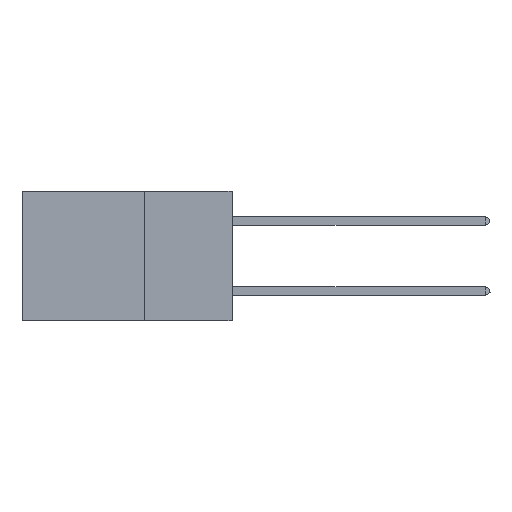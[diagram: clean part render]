
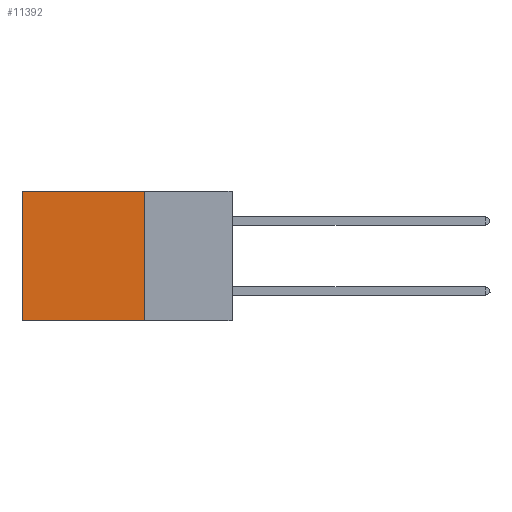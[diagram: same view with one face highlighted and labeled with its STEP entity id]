
A CAD part, left-side view. The second image highlights one B-rep face of the part: STEP entity #11392.
In plain terms, the highlighted planar face has unit normal (-1, 0, 0).
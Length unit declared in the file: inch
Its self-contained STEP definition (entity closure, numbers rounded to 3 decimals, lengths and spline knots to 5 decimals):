
#545 = CARTESIAN_POINT ( 'NONE',  ( 0.2875, 0.6, 0. ) ) ;
#556 = VERTEX_POINT ( 'NONE', #7631 ) ;
#778 = ORIENTED_EDGE ( 'NONE', *, *, #7028, .F. ) ;
#787 = EDGE_CURVE ( 'NONE', #556, #21670, #19484, .T. ) ;
#1865 = EDGE_CURVE ( 'NONE', #556, #8646, #19161, .T. ) ;
#1885 = VECTOR ( 'NONE', #12002, 39.37008 ) ;
#2304 = VERTEX_POINT ( 'NONE', #20187 ) ;
#3359 = AXIS2_PLACEMENT_3D ( 'NONE', #5498, #18232, #27047 ) ;
#5120 = EDGE_LOOP ( 'NONE', ( #17903, #778, #9570, #25273 ) ) ;
#5498 = CARTESIAN_POINT ( 'NONE',  ( 0.2875, 0.25, 0. ) ) ;
#7028 = EDGE_CURVE ( 'NONE', #8646, #2304, #26189, .T. ) ;
#7631 = CARTESIAN_POINT ( 'NONE',  ( 0.2875, 0.25, 0. ) ) ;
#7740 = VECTOR ( 'NONE', #9291, 39.37008 ) ;
#8248 = EDGE_CURVE ( 'NONE', #21670, #2304, #11084, .T. ) ;
#8646 = VERTEX_POINT ( 'NONE', #10606 ) ;
#9291 = DIRECTION ( 'NONE',  ( 0., 0., -1. ) ) ;
#9570 = ORIENTED_EDGE ( 'NONE', *, *, #1865, .F. ) ;
#10003 = CARTESIAN_POINT ( 'NONE',  ( 0.2875, 0.25, 0. ) ) ;
#10606 = CARTESIAN_POINT ( 'NONE',  ( 0.2875, 0.25, -0.37 ) ) ;
#11084 = LINE ( 'NONE', #18256, #1885 ) ;
#11392 = ADVANCED_FACE ( 'NONE', ( #13857 ), #24063, .F. ) ;
#12002 = DIRECTION ( 'NONE',  ( 0., 0., -1. ) ) ;
#13857 = FACE_OUTER_BOUND ( 'NONE', #5120, .T. ) ;
#13936 = VECTOR ( 'NONE', #15509, 39.37008 ) ;
#15509 = DIRECTION ( 'NONE',  ( 0., 1., 0. ) ) ;
#17903 = ORIENTED_EDGE ( 'NONE', *, *, #8248, .T. ) ;
#18232 = DIRECTION ( 'NONE',  ( 1., 0., 0. ) ) ;
#18256 = CARTESIAN_POINT ( 'NONE',  ( 0.2875, 0.6, 0. ) ) ;
#18484 = DIRECTION ( 'NONE',  ( 0., 1., 0. ) ) ;
#19161 = LINE ( 'NONE', #21252, #7740 ) ;
#19484 = LINE ( 'NONE', #10003, #13936 ) ;
#20187 = CARTESIAN_POINT ( 'NONE',  ( 0.2875, 0.6, -0.37 ) ) ;
#20311 = CARTESIAN_POINT ( 'NONE',  ( 0.2875, 0.25, -0.37 ) ) ;
#21252 = CARTESIAN_POINT ( 'NONE',  ( 0.2875, 0.25, 0. ) ) ;
#21670 = VERTEX_POINT ( 'NONE', #545 ) ;
#24063 = PLANE ( 'NONE',  #3359 ) ;
#25183 = VECTOR ( 'NONE', #18484, 39.37008 ) ;
#25273 = ORIENTED_EDGE ( 'NONE', *, *, #787, .T. ) ;
#26189 = LINE ( 'NONE', #20311, #25183 ) ;
#27047 = DIRECTION ( 'NONE',  ( 0., 0., -1. ) ) ;
